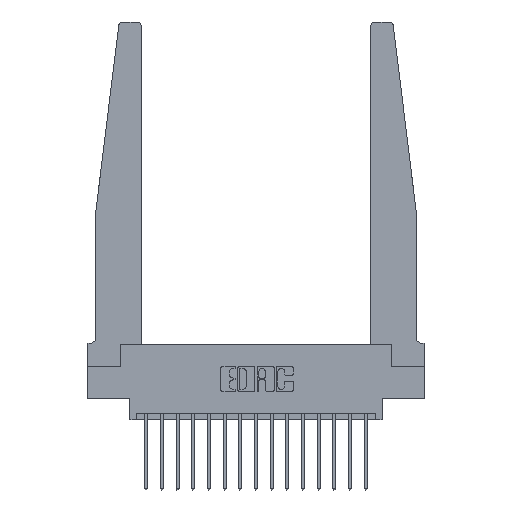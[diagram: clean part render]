
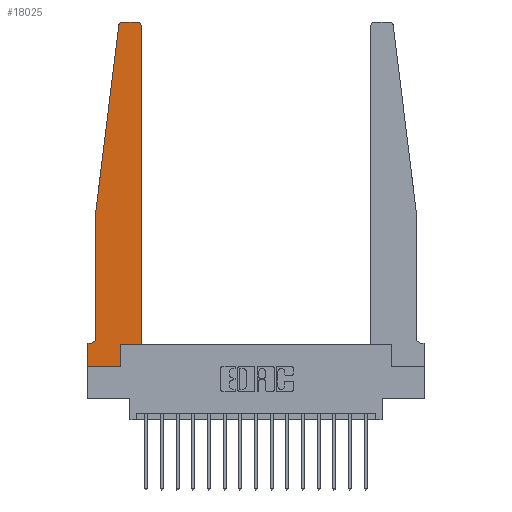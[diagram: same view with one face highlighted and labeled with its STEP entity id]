
A CAD part, top view. The second image highlights one B-rep face of the part: STEP entity #18025.
In plain terms, the highlighted planar face has unit normal (0, 0, 1).
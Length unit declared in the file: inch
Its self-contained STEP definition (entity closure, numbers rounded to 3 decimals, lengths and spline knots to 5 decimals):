
#29 = VECTOR ( 'NONE', #10529, 39.37008 ) ;
#263 = VERTEX_POINT ( 'NONE', #9001 ) ;
#572 = ORIENTED_EDGE ( 'NONE', *, *, #2729, .T. ) ;
#615 = DIRECTION ( 'NONE',  ( -1., 0., 0. ) ) ;
#636 = VECTOR ( 'NONE', #8638, 39.37008 ) ;
#763 = CARTESIAN_POINT ( 'NONE',  ( 0., 0.1875, 0.37 ) ) ;
#863 = VECTOR ( 'NONE', #615, 39.37008 ) ;
#883 = LINE ( 'NONE', #18286, #15209 ) ;
#884 = VERTEX_POINT ( 'NONE', #13438 ) ;
#1131 = DIRECTION ( 'NONE',  ( 1., 0., 0. ) ) ;
#1633 = CARTESIAN_POINT ( 'NONE',  ( 0.395, 2.72, 0.37 ) ) ;
#1823 = VERTEX_POINT ( 'NONE', #16027 ) ;
#2192 = DIRECTION ( 'NONE',  ( 0., 0., -1. ) ) ;
#2376 = DIRECTION ( 'NONE',  ( 1., 0., 0. ) ) ;
#2483 = EDGE_CURVE ( 'NONE', #884, #5881, #883, .T. ) ;
#2590 = VECTOR ( 'NONE', #18162, 39.37008 ) ;
#2729 = EDGE_CURVE ( 'NONE', #5881, #16918, #14464, .T. ) ;
#2835 = EDGE_CURVE ( 'NONE', #16918, #11605, #10317, .T. ) ;
#3088 = VERTEX_POINT ( 'NONE', #9880 ) ;
#3195 = AXIS2_PLACEMENT_3D ( 'NONE', #13683, #2192, #5014 ) ;
#3254 = EDGE_CURVE ( 'NONE', #9503, #3088, #16143, .T. ) ;
#3346 = EDGE_CURVE ( 'NONE', #3088, #3939, #3669, .T. ) ;
#3429 = CIRCLE ( 'NONE', #15893, 0.03 ) ;
#3555 = ORIENTED_EDGE ( 'NONE', *, *, #15211, .T. ) ;
#3615 = CARTESIAN_POINT ( 'NONE',  ( 0.065, 1.25, 0.37 ) ) ;
#3669 = LINE ( 'NONE', #4719, #29 ) ;
#3939 = VERTEX_POINT ( 'NONE', #12945 ) ;
#3950 = CARTESIAN_POINT ( 'NONE',  ( 0.27653, 2.72, 0.37 ) ) ;
#3965 = ORIENTED_EDGE ( 'NONE', *, *, #9484, .T. ) ;
#4678 = ORIENTED_EDGE ( 'NONE', *, *, #3346, .T. ) ;
#4687 = EDGE_CURVE ( 'NONE', #5118, #263, #3429, .T. ) ;
#4719 = CARTESIAN_POINT ( 'NONE',  ( 0., 0., 0.37 ) ) ;
#5014 = DIRECTION ( 'NONE',  ( -1., 0., 0. ) ) ;
#5016 = VERTEX_POINT ( 'NONE', #15018 ) ;
#5118 = VERTEX_POINT ( 'NONE', #6076 ) ;
#5126 = DIRECTION ( 'NONE',  ( 0., -1., 0. ) ) ;
#5284 = VECTOR ( 'NONE', #5126, 39.37008 ) ;
#5296 = FACE_OUTER_BOUND ( 'NONE', #13444, .T. ) ;
#5609 = AXIS2_PLACEMENT_3D ( 'NONE', #763, #12720, #2376 ) ;
#5881 = VERTEX_POINT ( 'NONE', #8007 ) ;
#6076 = CARTESIAN_POINT ( 'NONE',  ( 0.27653, 2.75, 0.37 ) ) ;
#6120 = ORIENTED_EDGE ( 'NONE', *, *, #2483, .T. ) ;
#6206 = VECTOR ( 'NONE', #11585, 39.37008 ) ;
#7465 = LINE ( 'NONE', #18345, #2590 ) ;
#7665 = CARTESIAN_POINT ( 'NONE',  ( 0.425, 2.72, 0.37 ) ) ;
#7740 = CIRCLE ( 'NONE', #3195, 0.05 ) ;
#7829 = LINE ( 'NONE', #13625, #863 ) ;
#7892 = ORIENTED_EDGE ( 'NONE', *, *, #4687, .T. ) ;
#8007 = CARTESIAN_POINT ( 'NONE',  ( 0.425, 0.18, 0.37 ) ) ;
#8638 = DIRECTION ( 'NONE',  ( 0., -1., 0. ) ) ;
#8643 = ORIENTED_EDGE ( 'NONE', *, *, #16604, .T. ) ;
#9001 = CARTESIAN_POINT ( 'NONE',  ( 0.24675, 2.72367, 0.37 ) ) ;
#9124 = EDGE_CURVE ( 'NONE', #5016, #1823, #10846, .T. ) ;
#9484 = EDGE_CURVE ( 'NONE', #1823, #11466, #7740, .T. ) ;
#9503 = VERTEX_POINT ( 'NONE', #17878 ) ;
#9594 = PLANE ( 'NONE',  #5609 ) ;
#9767 = DIRECTION ( 'NONE',  ( 0., 0., 1. ) ) ;
#9880 = CARTESIAN_POINT ( 'NONE',  ( 0., 0., 0.37 ) ) ;
#10317 = CIRCLE ( 'NONE', #17054, 0.03 ) ;
#10529 = DIRECTION ( 'NONE',  ( 1., 0., 0. ) ) ;
#10814 = CARTESIAN_POINT ( 'NONE',  ( 0.065, 1.25, 0.37 ) ) ;
#10846 = LINE ( 'NONE', #3615, #5284 ) ;
#10855 = DIRECTION ( 'NONE',  ( 1., 0., 0. ) ) ;
#11173 = CARTESIAN_POINT ( 'NONE',  ( 0.015, 0.1875, 0.37 ) ) ;
#11466 = VERTEX_POINT ( 'NONE', #11173 ) ;
#11585 = DIRECTION ( 'NONE',  ( -1., 0., 0. ) ) ;
#11589 = ORIENTED_EDGE ( 'NONE', *, *, #2835, .T. ) ;
#11605 = VERTEX_POINT ( 'NONE', #13072 ) ;
#11791 = ORIENTED_EDGE ( 'NONE', *, *, #16230, .T. ) ;
#11840 = VECTOR ( 'NONE', #17791, 39.37008 ) ;
#11865 = CARTESIAN_POINT ( 'NONE',  ( 0., 0., 0.37 ) ) ;
#11975 = CARTESIAN_POINT ( 'NONE',  ( 0.425, 0.18, 0.37 ) ) ;
#12657 = ORIENTED_EDGE ( 'NONE', *, *, #3254, .T. ) ;
#12720 = DIRECTION ( 'NONE',  ( 0., 0., 1. ) ) ;
#12924 = CARTESIAN_POINT ( 'NONE',  ( 0.065, 0.1875, 0.37 ) ) ;
#12945 = CARTESIAN_POINT ( 'NONE',  ( 0.2605, 0., 0.37 ) ) ;
#13072 = CARTESIAN_POINT ( 'NONE',  ( 0.395, 2.75, 0.37 ) ) ;
#13218 = DIRECTION ( 'NONE',  ( 0., 0., 1. ) ) ;
#13288 = EDGE_CURVE ( 'NONE', #11605, #5118, #7829, .T. ) ;
#13350 = ORIENTED_EDGE ( 'NONE', *, *, #9124, .T. ) ;
#13438 = CARTESIAN_POINT ( 'NONE',  ( 0.2605, 0.18, 0.37 ) ) ;
#13444 = EDGE_LOOP ( 'NONE', ( #14004, #7892, #3555, #13350, #3965, #11791, #12657, #4678, #8643, #6120, #572, #11589 ) ) ;
#13625 = CARTESIAN_POINT ( 'NONE',  ( 0.25, 2.75, 0.37 ) ) ;
#13683 = CARTESIAN_POINT ( 'NONE',  ( 0.015, 0.2375, 0.37 ) ) ;
#14004 = ORIENTED_EDGE ( 'NONE', *, *, #13288, .T. ) ;
#14464 = LINE ( 'NONE', #11975, #11840 ) ;
#14556 = DIRECTION ( 'NONE',  ( 1., 0., 0. ) ) ;
#15001 = LINE ( 'NONE', #10814, #16207 ) ;
#15018 = CARTESIAN_POINT ( 'NONE',  ( 0.065, 1.25, 0.37 ) ) ;
#15209 = VECTOR ( 'NONE', #10855, 39.37008 ) ;
#15211 = EDGE_CURVE ( 'NONE', #263, #5016, #15001, .T. ) ;
#15893 = AXIS2_PLACEMENT_3D ( 'NONE', #3950, #9767, #1131 ) ;
#16027 = CARTESIAN_POINT ( 'NONE',  ( 0.065, 0.2375, 0.37 ) ) ;
#16143 = LINE ( 'NONE', #11865, #636 ) ;
#16207 = VECTOR ( 'NONE', #16632, 39.37008 ) ;
#16230 = EDGE_CURVE ( 'NONE', #11466, #9503, #17685, .T. ) ;
#16604 = EDGE_CURVE ( 'NONE', #3939, #884, #7465, .T. ) ;
#16632 = DIRECTION ( 'NONE',  ( -0.122, -0.992, 0. ) ) ;
#16918 = VERTEX_POINT ( 'NONE', #7665 ) ;
#17054 = AXIS2_PLACEMENT_3D ( 'NONE', #1633, #13218, #14556 ) ;
#17685 = LINE ( 'NONE', #12924, #6206 ) ;
#17791 = DIRECTION ( 'NONE',  ( 0., 1., 0. ) ) ;
#17878 = CARTESIAN_POINT ( 'NONE',  ( 0., 0.1875, 0.37 ) ) ;
#18025 = ADVANCED_FACE ( 'NONE', ( #5296 ), #9594, .T. ) ;
#18162 = DIRECTION ( 'NONE',  ( 0., 1., 0. ) ) ;
#18286 = CARTESIAN_POINT ( 'NONE',  ( 0.425, 0.18, 0.37 ) ) ;
#18345 = CARTESIAN_POINT ( 'NONE',  ( 0.2605, 0.18, 0.37 ) ) ;
